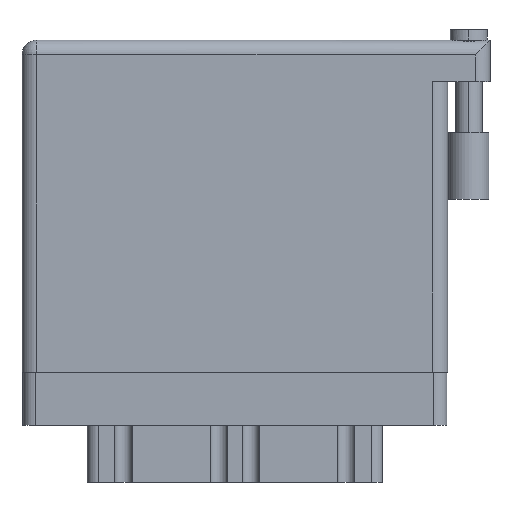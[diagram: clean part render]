
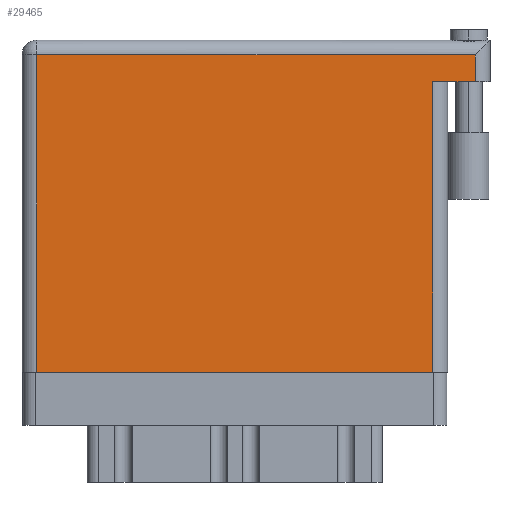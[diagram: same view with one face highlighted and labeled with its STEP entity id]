
A CAD part, front view. The second image highlights one B-rep face of the part: STEP entity #29465.
In plain terms, the highlighted face is planar.
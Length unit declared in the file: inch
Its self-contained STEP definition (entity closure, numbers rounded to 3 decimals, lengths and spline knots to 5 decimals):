
#194 = CARTESIAN_POINT ( 'NONE',  ( 0., 1.496, 0. ) ) ;
#590 = CARTESIAN_POINT ( 'NONE',  ( 0.07, 1.496, 0. ) ) ;
#776 = VERTEX_POINT ( 'NONE', #15885 ) ;
#913 = DIRECTION ( 'NONE',  ( 0., 1., 0. ) ) ;
#1030 = VERTEX_POINT ( 'NONE', #10446 ) ;
#1976 = CARTESIAN_POINT ( 'NONE',  ( 0.07, 0., 0. ) ) ;
#2113 = CARTESIAN_POINT ( 'NONE',  ( 2.138, 1.369, 0. ) ) ;
#2332 = VECTOR ( 'NONE', #21383, 39.37008 ) ;
#2373 = VERTEX_POINT ( 'NONE', #2113 ) ;
#2512 = CARTESIAN_POINT ( 'NONE',  ( 1.938, 1.369, 0. ) ) ;
#2965 = CARTESIAN_POINT ( 'NONE',  ( 1.938, 0., 0. ) ) ;
#4288 = DIRECTION ( 'NONE',  ( -1., 0., 0. ) ) ;
#4315 = DIRECTION ( 'NONE',  ( -1., 0., 0. ) ) ;
#4528 = DIRECTION ( 'NONE',  ( -1., 0., 0. ) ) ;
#4561 = CARTESIAN_POINT ( 'NONE',  ( 0., 0., 0. ) ) ;
#5832 = VERTEX_POINT ( 'NONE', #10526 ) ;
#6032 = CARTESIAN_POINT ( 'NONE',  ( 0., 1.566, 0. ) ) ;
#7695 = CARTESIAN_POINT ( 'NONE',  ( 2.138, 1.566, 0. ) ) ;
#10063 = EDGE_LOOP ( 'NONE', ( #29060, #10880, #14006, #12774, #27972, #27446 ) ) ;
#10446 = CARTESIAN_POINT ( 'NONE',  ( 1.938, 1.369, 0. ) ) ;
#10526 = CARTESIAN_POINT ( 'NONE',  ( 0.07, 0., 0. ) ) ;
#10880 = ORIENTED_EDGE ( 'NONE', *, *, #13227, .T. ) ;
#11927 = DIRECTION ( 'NONE',  ( 0., 1., 0. ) ) ;
#12774 = ORIENTED_EDGE ( 'NONE', *, *, #15455, .T. ) ;
#12983 = FACE_OUTER_BOUND ( 'NONE', #10063, .T. ) ;
#13227 = EDGE_CURVE ( 'NONE', #13347, #1030, #14239, .T. ) ;
#13347 = VERTEX_POINT ( 'NONE', #2965 ) ;
#14006 = ORIENTED_EDGE ( 'NONE', *, *, #16885, .F. ) ;
#14239 = LINE ( 'NONE', #2512, #21197 ) ;
#14284 = VECTOR ( 'NONE', #913, 39.37008 ) ;
#15455 = EDGE_CURVE ( 'NONE', #2373, #776, #17743, .T. ) ;
#15885 = CARTESIAN_POINT ( 'NONE',  ( 2.138, 1.496, 0. ) ) ;
#15933 = VERTEX_POINT ( 'NONE', #590 ) ;
#16271 = VECTOR ( 'NONE', #20348, 39.37008 ) ;
#16316 = VECTOR ( 'NONE', #4288, 39.37008 ) ;
#16885 = EDGE_CURVE ( 'NONE', #2373, #1030, #27770, .T. ) ;
#17743 = LINE ( 'NONE', #7695, #14284 ) ;
#17839 = EDGE_CURVE ( 'NONE', #776, #15933, #25696, .T. ) ;
#19216 = LINE ( 'NONE', #4561, #2332 ) ;
#20348 = DIRECTION ( 'NONE',  ( 0., -1., 0. ) ) ;
#21197 = VECTOR ( 'NONE', #11927, 39.37008 ) ;
#21256 = AXIS2_PLACEMENT_3D ( 'NONE', #6032, #25482, #4315 ) ;
#21383 = DIRECTION ( 'NONE',  ( 1., 0., 0. ) ) ;
#21540 = EDGE_CURVE ( 'NONE', #5832, #13347, #19216, .T. ) ;
#22403 = PLANE ( 'NONE',  #21256 ) ;
#23125 = LINE ( 'NONE', #1976, #16271 ) ;
#24630 = VECTOR ( 'NONE', #4528, 39.37008 ) ;
#25453 = CARTESIAN_POINT ( 'NONE',  ( 2.208, 1.369, 0. ) ) ;
#25482 = DIRECTION ( 'NONE',  ( 0., 0., -1. ) ) ;
#25696 = LINE ( 'NONE', #194, #24630 ) ;
#27446 = ORIENTED_EDGE ( 'NONE', *, *, #28737, .T. ) ;
#27770 = LINE ( 'NONE', #25453, #16316 ) ;
#27972 = ORIENTED_EDGE ( 'NONE', *, *, #17839, .T. ) ;
#28737 = EDGE_CURVE ( 'NONE', #15933, #5832, #23125, .T. ) ;
#29060 = ORIENTED_EDGE ( 'NONE', *, *, #21540, .T. ) ;
#29465 = ADVANCED_FACE ( 'NONE', ( #12983 ), #22403, .F. ) ;
